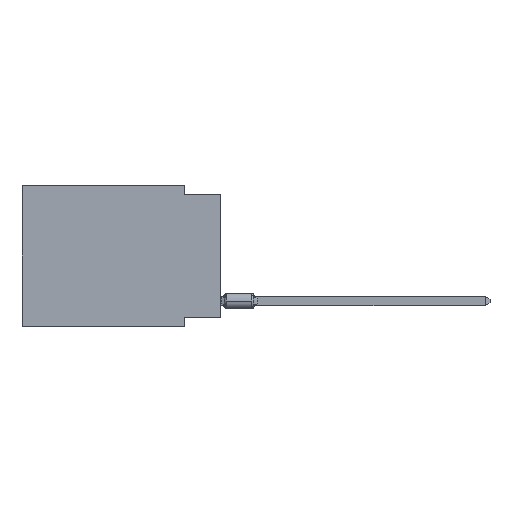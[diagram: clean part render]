
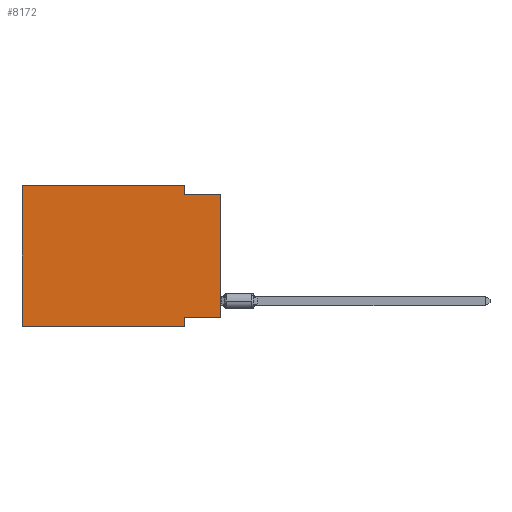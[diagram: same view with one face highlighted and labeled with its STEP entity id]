
A CAD part, left-side view. The second image highlights one B-rep face of the part: STEP entity #8172.
In plain terms, the highlighted planar face has unit normal (-1, 0, 0).
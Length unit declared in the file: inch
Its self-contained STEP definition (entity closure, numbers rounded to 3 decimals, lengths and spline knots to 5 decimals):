
#176 = VERTEX_POINT ( 'NONE', #14993 ) ;
#1952 = EDGE_CURVE ( 'NONE', #29202, #36999, #19963, .T. ) ;
#2516 = CARTESIAN_POINT ( 'NONE',  ( 0., 0., -0.365 ) ) ;
#4558 = VECTOR ( 'NONE', #27660, 39.37008 ) ;
#5453 = DIRECTION ( 'NONE',  ( 0., 1., 0. ) ) ;
#6229 = EDGE_CURVE ( 'NONE', #29202, #31967, #22336, .T. ) ;
#6634 = ORIENTED_EDGE ( 'NONE', *, *, #18107, .F. ) ;
#6823 = DIRECTION ( 'NONE',  ( 0., 0., -1. ) ) ;
#6943 = CARTESIAN_POINT ( 'NONE',  ( 0., 0.55, 0. ) ) ;
#7042 = VERTEX_POINT ( 'NONE', #30205 ) ;
#7238 = CARTESIAN_POINT ( 'NONE',  ( 0., 0.1, 0. ) ) ;
#8172 = ADVANCED_FACE ( 'NONE', ( #25054 ), #18530, .F. ) ;
#9188 = VECTOR ( 'NONE', #5453, 39.37008 ) ;
#9910 = CARTESIAN_POINT ( 'NONE',  ( 0., 0., -0.025 ) ) ;
#11766 = CARTESIAN_POINT ( 'NONE',  ( 0., 0.1, -0.025 ) ) ;
#11860 = VERTEX_POINT ( 'NONE', #9910 ) ;
#12267 = DIRECTION ( 'NONE',  ( 0., -1., 0. ) ) ;
#12655 = ORIENTED_EDGE ( 'NONE', *, *, #1952, .F. ) ;
#12710 = LINE ( 'NONE', #31187, #41043 ) ;
#12723 = DIRECTION ( 'NONE',  ( 0., 0., -1. ) ) ;
#12882 = EDGE_CURVE ( 'NONE', #176, #11860, #36732, .T. ) ;
#13591 = CARTESIAN_POINT ( 'NONE',  ( 0., 0.55, 0. ) ) ;
#14442 = CARTESIAN_POINT ( 'NONE',  ( 0., 0., 0. ) ) ;
#14845 = CARTESIAN_POINT ( 'NONE',  ( 0., 0., -0.025 ) ) ;
#14993 = CARTESIAN_POINT ( 'NONE',  ( 0., 0., -0.365 ) ) ;
#15124 = VECTOR ( 'NONE', #16606, 39.37008 ) ;
#15647 = EDGE_CURVE ( 'NONE', #7042, #31967, #28055, .T. ) ;
#16606 = DIRECTION ( 'NONE',  ( 0., 0., 1. ) ) ;
#16792 = ORIENTED_EDGE ( 'NONE', *, *, #17141, .F. ) ;
#17141 = EDGE_CURVE ( 'NONE', #35726, #23326, #35613, .T. ) ;
#17489 = CARTESIAN_POINT ( 'NONE',  ( 0., 0.55, -0.39 ) ) ;
#17792 = LINE ( 'NONE', #14845, #4558 ) ;
#17950 = VECTOR ( 'NONE', #12267, 39.37008 ) ;
#18107 = EDGE_CURVE ( 'NONE', #23326, #11860, #17792, .T. ) ;
#18383 = DIRECTION ( 'NONE',  ( 0., -1., 0. ) ) ;
#18530 = PLANE ( 'NONE',  #38607 ) ;
#18594 = EDGE_LOOP ( 'NONE', ( #30865, #6634, #16792, #31109, #12655, #32525, #29976, #21629 ) ) ;
#18823 = CARTESIAN_POINT ( 'NONE',  ( 0., 0.1, -0.39 ) ) ;
#19963 = LINE ( 'NONE', #6943, #15124 ) ;
#21629 = ORIENTED_EDGE ( 'NONE', *, *, #35602, .F. ) ;
#22336 = LINE ( 'NONE', #31994, #17950 ) ;
#22424 = EDGE_CURVE ( 'NONE', #36999, #35726, #12710, .T. ) ;
#23326 = VERTEX_POINT ( 'NONE', #11766 ) ;
#25054 = FACE_OUTER_BOUND ( 'NONE', #18594, .T. ) ;
#25296 = CARTESIAN_POINT ( 'NONE',  ( 0., 0.1, -0.39 ) ) ;
#25332 = VECTOR ( 'NONE', #6823, 39.37008 ) ;
#27660 = DIRECTION ( 'NONE',  ( 0., -1., 0. ) ) ;
#28055 = LINE ( 'NONE', #18823, #29095 ) ;
#29095 = VECTOR ( 'NONE', #12723, 39.37008 ) ;
#29202 = VERTEX_POINT ( 'NONE', #17489 ) ;
#29976 = ORIENTED_EDGE ( 'NONE', *, *, #15647, .F. ) ;
#30205 = CARTESIAN_POINT ( 'NONE',  ( 0., 0.1, -0.365 ) ) ;
#30865 = ORIENTED_EDGE ( 'NONE', *, *, #12882, .T. ) ;
#31109 = ORIENTED_EDGE ( 'NONE', *, *, #22424, .F. ) ;
#31187 = CARTESIAN_POINT ( 'NONE',  ( 0., 0.55, 0. ) ) ;
#31720 = LINE ( 'NONE', #2516, #9188 ) ;
#31831 = VECTOR ( 'NONE', #39870, 39.37008 ) ;
#31967 = VERTEX_POINT ( 'NONE', #25296 ) ;
#31994 = CARTESIAN_POINT ( 'NONE',  ( 0., 0.55, -0.39 ) ) ;
#32525 = ORIENTED_EDGE ( 'NONE', *, *, #6229, .T. ) ;
#34502 = DIRECTION ( 'NONE',  ( 0., 0., -1. ) ) ;
#34930 = CARTESIAN_POINT ( 'NONE',  ( 0., 0.55, 0. ) ) ;
#35084 = CARTESIAN_POINT ( 'NONE',  ( 0., 0.1, 0. ) ) ;
#35602 = EDGE_CURVE ( 'NONE', #176, #7042, #31720, .T. ) ;
#35613 = LINE ( 'NONE', #7238, #25332 ) ;
#35726 = VERTEX_POINT ( 'NONE', #35084 ) ;
#36732 = LINE ( 'NONE', #14442, #31831 ) ;
#36999 = VERTEX_POINT ( 'NONE', #13591 ) ;
#37870 = DIRECTION ( 'NONE',  ( 1., 0., 0. ) ) ;
#38607 = AXIS2_PLACEMENT_3D ( 'NONE', #34930, #37870, #34502 ) ;
#39870 = DIRECTION ( 'NONE',  ( 0., 0., 1. ) ) ;
#41043 = VECTOR ( 'NONE', #18383, 39.37008 ) ;
